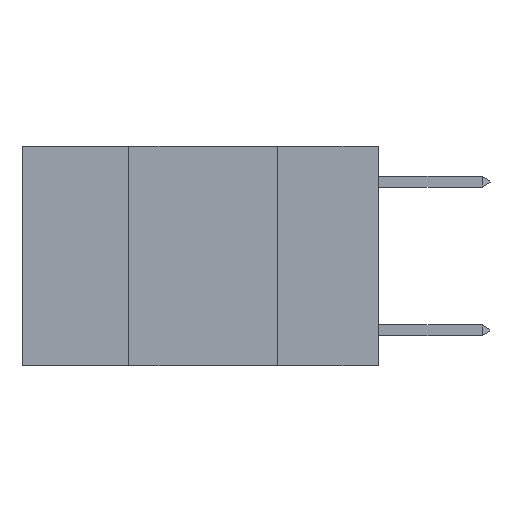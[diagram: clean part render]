
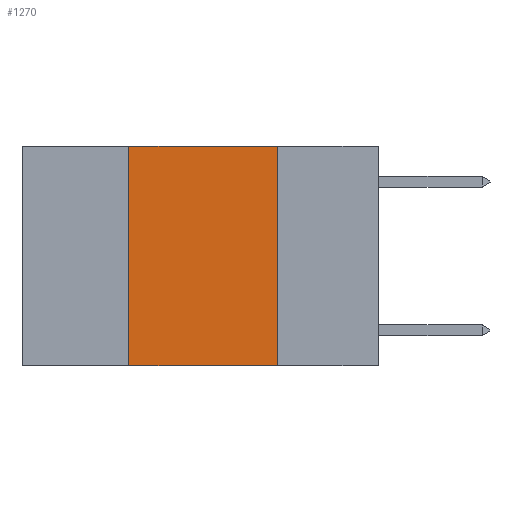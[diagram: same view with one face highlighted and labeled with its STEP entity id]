
A CAD part, left-side view. The second image highlights one B-rep face of the part: STEP entity #1270.
In plain terms, the highlighted planar face has unit normal (-1, 0, 0).
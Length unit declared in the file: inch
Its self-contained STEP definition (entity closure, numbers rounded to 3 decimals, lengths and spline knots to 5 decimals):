
#151 = CARTESIAN_POINT ( 'NONE',  ( 0., 0.42, -0.37 ) ) ;
#222 = DIRECTION ( 'NONE',  ( 0., 0., -1. ) ) ;
#344 = CARTESIAN_POINT ( 'NONE',  ( 0., 0.42, 0. ) ) ;
#485 = CARTESIAN_POINT ( 'NONE',  ( 0., 0.6, 0. ) ) ;
#972 = VERTEX_POINT ( 'NONE', #151 ) ;
#1091 = DIRECTION ( 'NONE',  ( 0., 0., 1. ) ) ;
#1247 = ORIENTED_EDGE ( 'NONE', *, *, #7371, .T. ) ;
#1260 = EDGE_CURVE ( 'NONE', #3192, #3850, #4734, .T. ) ;
#1270 = ADVANCED_FACE ( 'NONE', ( #6492 ), #7981, .F. ) ;
#1400 = ORIENTED_EDGE ( 'NONE', *, *, #1260, .F. ) ;
#1932 = VERTEX_POINT ( 'NONE', #3917 ) ;
#2089 = LINE ( 'NONE', #344, #5636 ) ;
#2953 = CARTESIAN_POINT ( 'NONE',  ( 0., 0.42, 0. ) ) ;
#3192 = VERTEX_POINT ( 'NONE', #2953 ) ;
#3356 = VECTOR ( 'NONE', #222, 39.37008 ) ;
#3492 = CARTESIAN_POINT ( 'NONE',  ( 0., 0.6, -0.37 ) ) ;
#3850 = VERTEX_POINT ( 'NONE', #6750 ) ;
#3917 = CARTESIAN_POINT ( 'NONE',  ( 0., 0.17, -0.37 ) ) ;
#4048 = AXIS2_PLACEMENT_3D ( 'NONE', #7189, #8739, #4241 ) ;
#4241 = DIRECTION ( 'NONE',  ( 0., 0., -1. ) ) ;
#4261 = VECTOR ( 'NONE', #7207, 39.37008 ) ;
#4728 = CARTESIAN_POINT ( 'NONE',  ( 0., 0.17, 0. ) ) ;
#4734 = LINE ( 'NONE', #485, #4261 ) ;
#5636 = VECTOR ( 'NONE', #1091, 39.37008 ) ;
#6095 = EDGE_LOOP ( 'NONE', ( #6570, #1400, #6847, #1247 ) ) ;
#6224 = VECTOR ( 'NONE', #8752, 39.37008 ) ;
#6492 = FACE_OUTER_BOUND ( 'NONE', #6095, .T. ) ;
#6570 = ORIENTED_EDGE ( 'NONE', *, *, #9138, .F. ) ;
#6750 = CARTESIAN_POINT ( 'NONE',  ( 0., 0.17, 0. ) ) ;
#6847 = ORIENTED_EDGE ( 'NONE', *, *, #7232, .F. ) ;
#7189 = CARTESIAN_POINT ( 'NONE',  ( 0., 0.6, 0. ) ) ;
#7207 = DIRECTION ( 'NONE',  ( 0., -1., 0. ) ) ;
#7232 = EDGE_CURVE ( 'NONE', #972, #3192, #2089, .T. ) ;
#7340 = LINE ( 'NONE', #4728, #3356 ) ;
#7371 = EDGE_CURVE ( 'NONE', #972, #1932, #8220, .T. ) ;
#7981 = PLANE ( 'NONE',  #4048 ) ;
#8220 = LINE ( 'NONE', #3492, #6224 ) ;
#8739 = DIRECTION ( 'NONE',  ( 1., 0., 0. ) ) ;
#8752 = DIRECTION ( 'NONE',  ( 0., -1., 0. ) ) ;
#9138 = EDGE_CURVE ( 'NONE', #3850, #1932, #7340, .T. ) ;
